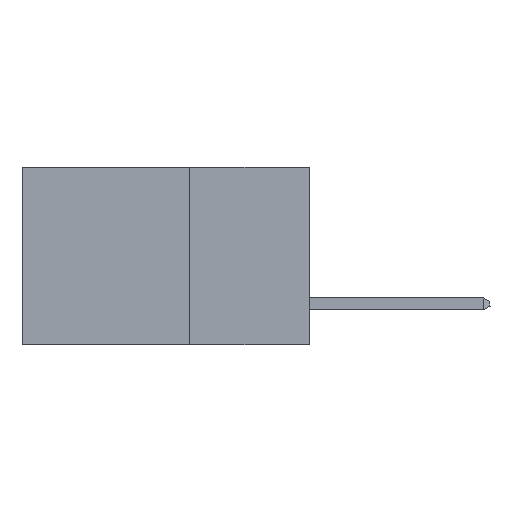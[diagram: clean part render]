
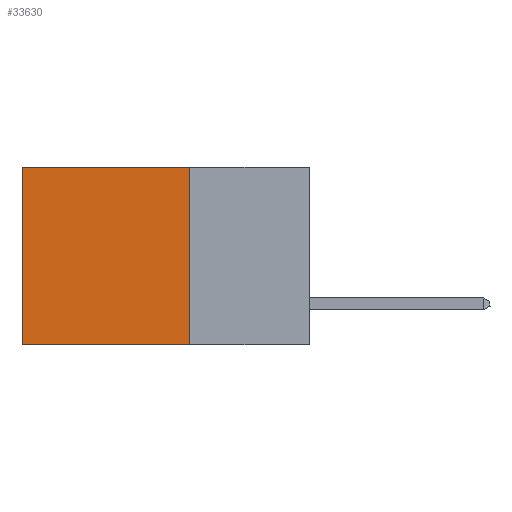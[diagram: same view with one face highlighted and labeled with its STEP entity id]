
A CAD part, left-side view. The second image highlights one B-rep face of the part: STEP entity #33630.
In plain terms, the highlighted planar face has unit normal (-1, 0, 0).
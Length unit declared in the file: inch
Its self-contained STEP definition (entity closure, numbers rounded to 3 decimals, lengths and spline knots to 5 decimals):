
#252 = DIRECTION ( 'NONE',  ( 0., 0., -1. ) ) ;
#1766 = ORIENTED_EDGE ( 'NONE', *, *, #13535, .F. ) ;
#2323 = CARTESIAN_POINT ( 'NONE',  ( 0.2875, 0.25, -0.37 ) ) ;
#6042 = CARTESIAN_POINT ( 'NONE',  ( 0.2875, 0.25, 0. ) ) ;
#6112 = LINE ( 'NONE', #13243, #33852 ) ;
#6964 = VERTEX_POINT ( 'NONE', #8352 ) ;
#8352 = CARTESIAN_POINT ( 'NONE',  ( 0.2875, 0.25, 0. ) ) ;
#10076 = CARTESIAN_POINT ( 'NONE',  ( 0.2875, 0.25, -0.37 ) ) ;
#10099 = VERTEX_POINT ( 'NONE', #17588 ) ;
#10936 = AXIS2_PLACEMENT_3D ( 'NONE', #6042, #30958, #14515 ) ;
#13243 = CARTESIAN_POINT ( 'NONE',  ( 0.2875, 0.6, 0. ) ) ;
#13535 = EDGE_CURVE ( 'NONE', #21282, #31622, #31808, .T. ) ;
#14515 = DIRECTION ( 'NONE',  ( 0., 0., -1. ) ) ;
#15851 = CARTESIAN_POINT ( 'NONE',  ( 0.2875, 0.6, -0.37 ) ) ;
#16664 = LINE ( 'NONE', #28175, #29841 ) ;
#17588 = CARTESIAN_POINT ( 'NONE',  ( 0.2875, 0.6, 0. ) ) ;
#19869 = PLANE ( 'NONE',  #10936 ) ;
#21282 = VERTEX_POINT ( 'NONE', #2323 ) ;
#24557 = VECTOR ( 'NONE', #31531, 39.37008 ) ;
#25071 = DIRECTION ( 'NONE',  ( 0., 1., 0. ) ) ;
#25388 = FACE_OUTER_BOUND ( 'NONE', #31463, .T. ) ;
#27758 = EDGE_CURVE ( 'NONE', #6964, #10099, #16664, .T. ) ;
#28000 = ORIENTED_EDGE ( 'NONE', *, *, #33478, .T. ) ;
#28175 = CARTESIAN_POINT ( 'NONE',  ( 0.2875, 0.25, 0. ) ) ;
#28889 = ORIENTED_EDGE ( 'NONE', *, *, #29440, .F. ) ;
#29440 = EDGE_CURVE ( 'NONE', #6964, #21282, #30744, .T. ) ;
#29841 = VECTOR ( 'NONE', #25071, 39.37008 ) ;
#29892 = VECTOR ( 'NONE', #33980, 39.37008 ) ;
#30744 = LINE ( 'NONE', #31485, #29892 ) ;
#30958 = DIRECTION ( 'NONE',  ( 1., 0., 0. ) ) ;
#31070 = ORIENTED_EDGE ( 'NONE', *, *, #27758, .T. ) ;
#31463 = EDGE_LOOP ( 'NONE', ( #28000, #1766, #28889, #31070 ) ) ;
#31485 = CARTESIAN_POINT ( 'NONE',  ( 0.2875, 0.25, 0. ) ) ;
#31531 = DIRECTION ( 'NONE',  ( 0., 1., 0. ) ) ;
#31622 = VERTEX_POINT ( 'NONE', #15851 ) ;
#31808 = LINE ( 'NONE', #10076, #24557 ) ;
#33478 = EDGE_CURVE ( 'NONE', #10099, #31622, #6112, .T. ) ;
#33630 = ADVANCED_FACE ( 'NONE', ( #25388 ), #19869, .F. ) ;
#33852 = VECTOR ( 'NONE', #252, 39.37008 ) ;
#33980 = DIRECTION ( 'NONE',  ( 0., 0., -1. ) ) ;
